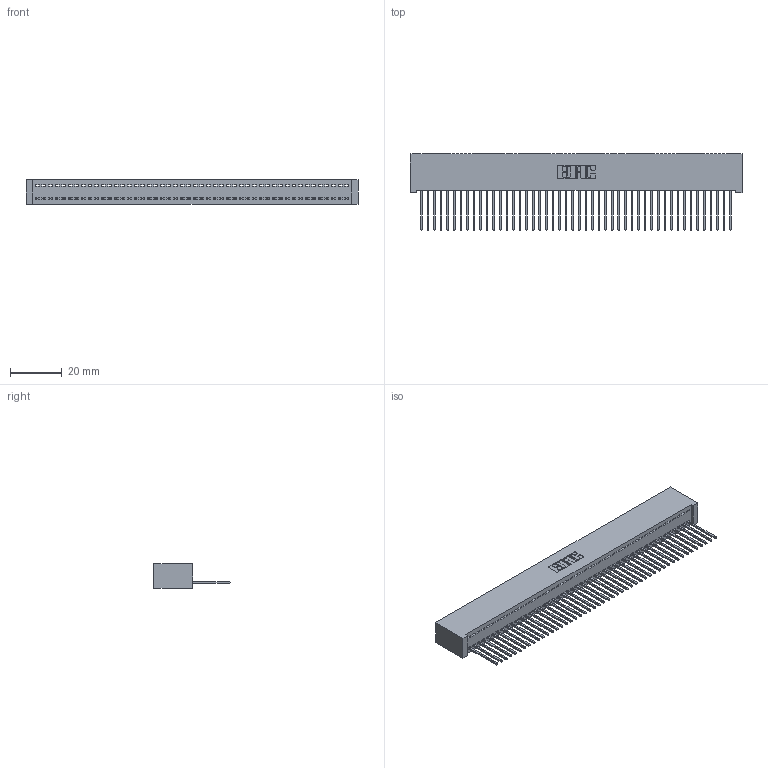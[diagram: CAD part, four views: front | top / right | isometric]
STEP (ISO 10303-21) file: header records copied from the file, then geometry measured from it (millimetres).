
FILE_DESCRIPTION (( 'STEP AP203' ), '1' );
FILE_NAME ('392-048-540-101.STEP', '2019-10-08T01:00:15', ( '' ), ( '' ), 'SwSTEP 2.0', 'SolidWorks 2016', '' );
FILE_SCHEMA (( 'CONFIG_CONTROL_DESIGN' ));
Length unit declared in the file: inch
Products named in the file (3): 345-292-001_345-293-140; 392-048-540-101; 342 Part_Lugless
Assembly tree (49 placements, depth 2):
  392-048-540-101
    342 Part_Lugless
    345-292-001_345-293-140  x48
Bounding box: 128.17 x 29.47 x 9.4 mm (x, y, z)
Volume: 11733.9 mm3; surface area: 18115.5 mm2
Topology: 49 solids, 49 shells, 2886 faces, 8723 edges, 5750 vertices
Faces by surface type: plane 2078, cylinder 808
Entity records: 28177 total; most frequent: CARTESIAN_POINT 4866, ORIENTED_EDGE 4850, DIRECTION 4085, EDGE_CURVE 2425, LINE 2305, VECTOR 2305, VERTEX_POINT 1614, AXIS2_PLACEMENT_3D 890
